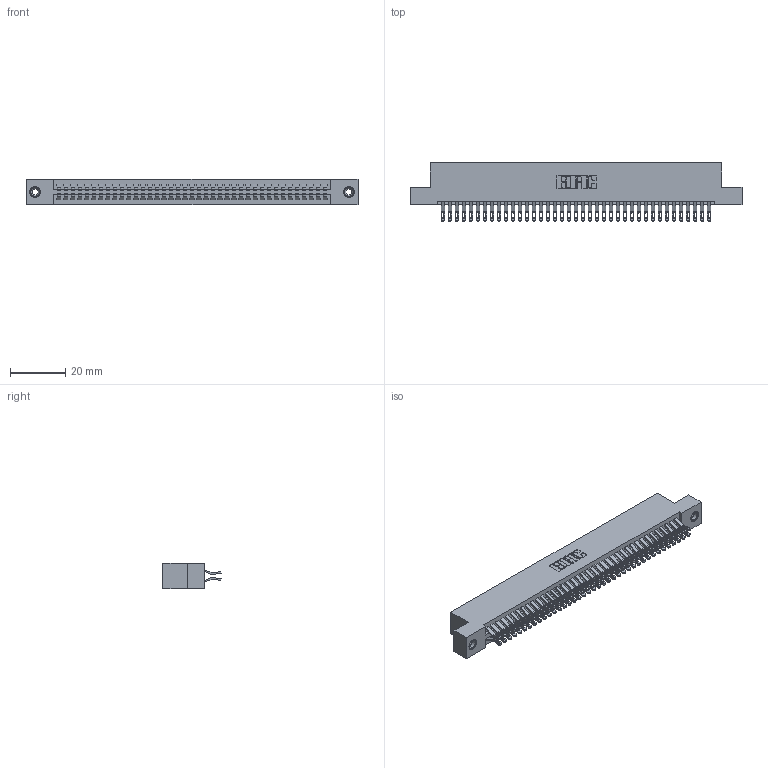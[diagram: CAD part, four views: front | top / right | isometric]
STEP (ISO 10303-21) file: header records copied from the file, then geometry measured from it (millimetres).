
FILE_DESCRIPTION (( 'STEP AP203' ), '1' );
FILE_NAME ('395-078-555-208.STEP', '2019-10-25T02:51:16', ( '' ), ( '' ), 'SwSTEP 2.0', 'SolidWorks 2016', '' );
FILE_SCHEMA (( 'CONFIG_CONTROL_DESIGN' ));
Length unit declared in the file: inch
Products named in the file (4): 345 Part_Flush Mounting Lugs - 0.156 Dia-TI; 345-292-001_555 Tail; 345-250-001_345-250-003-102; 395-078-555-208
Assembly tree (81 placements, depth 2):
  395-078-555-208
    345 Part_Flush Mounting Lugs - 0.156 Dia-TI
    345-292-001_555 Tail  x78
    345-250-001_345-250-003-102  x2
Bounding box: 120.27 x 21.13 x 9.4 mm (x, y, z)
Volume: 11874.9 mm3; surface area: 18295.4 mm2
Topology: 81 solids, 81 shells, 4554 faces, 14283 edges, 9514 vertices
Faces by surface type: plane 2530, cylinder 2008, cone 12, torus 4
Entity records: 32516 total; most frequent: CARTESIAN_POINT 5469, ORIENTED_EDGE 5366, DIRECTION 4821, EDGE_CURVE 2683, VECTOR 2355, LINE 2355, VERTEX_POINT 1784, AXIS2_PLACEMENT_3D 1233
